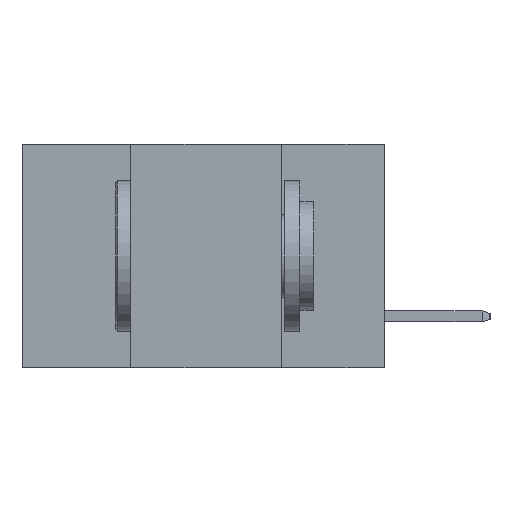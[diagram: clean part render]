
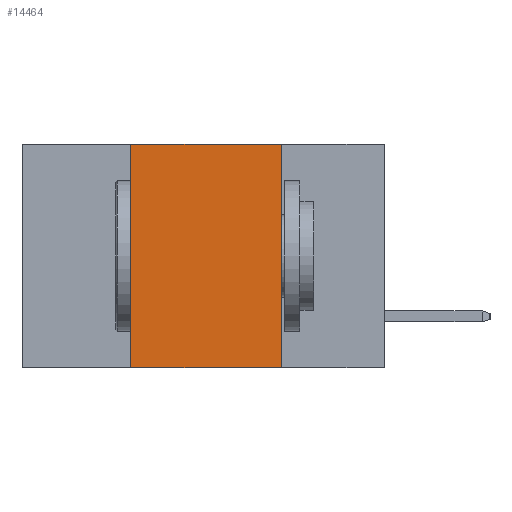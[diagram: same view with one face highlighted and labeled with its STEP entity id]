
A CAD part, left-side view. The second image highlights one B-rep face of the part: STEP entity #14464.
In plain terms, the highlighted planar face has unit normal (-1, 0, 0).
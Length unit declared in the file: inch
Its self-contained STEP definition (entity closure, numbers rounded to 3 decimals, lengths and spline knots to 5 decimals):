
#1300 = DIRECTION ( 'NONE',  ( 0., 0., -1. ) ) ;
#1358 = VERTEX_POINT ( 'NONE', #7556 ) ;
#1515 = EDGE_CURVE ( 'NONE', #1358, #18997, #19453, .T. ) ;
#3196 = CARTESIAN_POINT ( 'NONE',  ( 0., 0.6, 0. ) ) ;
#4825 = VECTOR ( 'NONE', #1300, 39.37008 ) ;
#6575 = EDGE_CURVE ( 'NONE', #18997, #24806, #8342, .T. ) ;
#6763 = ORIENTED_EDGE ( 'NONE', *, *, #1515, .F. ) ;
#7404 = CARTESIAN_POINT ( 'NONE',  ( 0., 0.42, 0. ) ) ;
#7553 = PLANE ( 'NONE',  #9335 ) ;
#7556 = CARTESIAN_POINT ( 'NONE',  ( 0., 0.42, -0.37 ) ) ;
#8342 = LINE ( 'NONE', #24307, #18776 ) ;
#9126 = DIRECTION ( 'NONE',  ( 0., 0., 1. ) ) ;
#9335 = AXIS2_PLACEMENT_3D ( 'NONE', #3196, #9644, #24214 ) ;
#9644 = DIRECTION ( 'NONE',  ( 1., 0., 0. ) ) ;
#11815 = CARTESIAN_POINT ( 'NONE',  ( 0., 0.17, 0. ) ) ;
#12959 = EDGE_CURVE ( 'NONE', #1358, #17831, #14951, .T. ) ;
#13970 = CARTESIAN_POINT ( 'NONE',  ( 0., 0.17, -0.37 ) ) ;
#14464 = ADVANCED_FACE ( 'NONE', ( #17464 ), #7553, .F. ) ;
#14951 = LINE ( 'NONE', #27152, #20491 ) ;
#16959 = DIRECTION ( 'NONE',  ( 0., -1., 0. ) ) ;
#17464 = FACE_OUTER_BOUND ( 'NONE', #23864, .T. ) ;
#17831 = VERTEX_POINT ( 'NONE', #13970 ) ;
#17892 = ORIENTED_EDGE ( 'NONE', *, *, #12959, .T. ) ;
#18776 = VECTOR ( 'NONE', #24236, 39.37008 ) ;
#18997 = VERTEX_POINT ( 'NONE', #7404 ) ;
#19453 = LINE ( 'NONE', #23661, #24912 ) ;
#20491 = VECTOR ( 'NONE', #16959, 39.37008 ) ;
#21018 = EDGE_CURVE ( 'NONE', #24806, #17831, #21600, .T. ) ;
#21489 = ORIENTED_EDGE ( 'NONE', *, *, #21018, .F. ) ;
#21600 = LINE ( 'NONE', #22352, #4825 ) ;
#22119 = ORIENTED_EDGE ( 'NONE', *, *, #6575, .F. ) ;
#22352 = CARTESIAN_POINT ( 'NONE',  ( 0., 0.17, 0. ) ) ;
#23661 = CARTESIAN_POINT ( 'NONE',  ( 0., 0.42, 0. ) ) ;
#23864 = EDGE_LOOP ( 'NONE', ( #21489, #22119, #6763, #17892 ) ) ;
#24214 = DIRECTION ( 'NONE',  ( 0., 0., -1. ) ) ;
#24236 = DIRECTION ( 'NONE',  ( 0., -1., 0. ) ) ;
#24307 = CARTESIAN_POINT ( 'NONE',  ( 0., 0.6, 0. ) ) ;
#24806 = VERTEX_POINT ( 'NONE', #11815 ) ;
#24912 = VECTOR ( 'NONE', #9126, 39.37008 ) ;
#27152 = CARTESIAN_POINT ( 'NONE',  ( 0., 0.6, -0.37 ) ) ;
